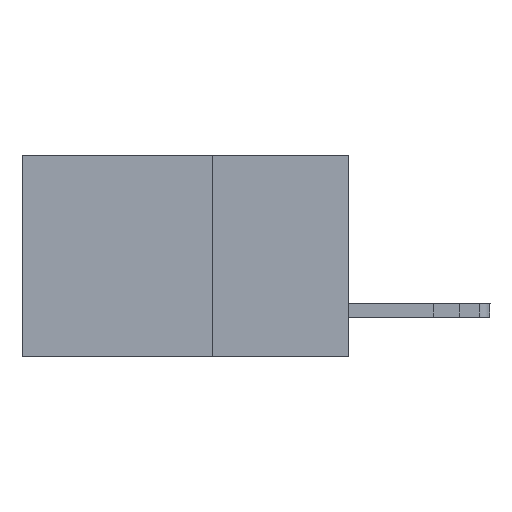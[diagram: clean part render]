
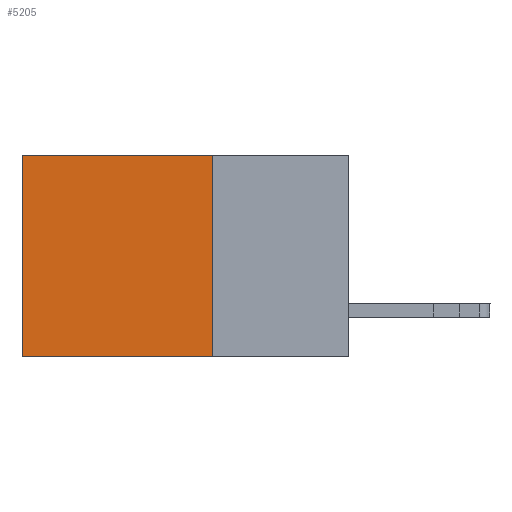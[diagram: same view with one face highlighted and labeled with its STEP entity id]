
A CAD part, left-side view. The second image highlights one B-rep face of the part: STEP entity #5205.
In plain terms, the highlighted planar face has unit normal (-1, 0, 0).
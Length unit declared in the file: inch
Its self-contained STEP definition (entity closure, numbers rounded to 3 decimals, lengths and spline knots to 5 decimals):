
#252 = EDGE_CURVE ( 'NONE', #12059, #4546, #9393, .T. ) ;
#828 = CARTESIAN_POINT ( 'NONE',  ( 0.2615, 0.25, 0. ) ) ;
#1049 = VECTOR ( 'NONE', #12565, 39.37008 ) ;
#1691 = CARTESIAN_POINT ( 'NONE',  ( 0.2615, 0.6, -0.37 ) ) ;
#1848 = EDGE_CURVE ( 'NONE', #4728, #4546, #3767, .T. ) ;
#2175 = CARTESIAN_POINT ( 'NONE',  ( 0.2615, 0.25, -0.37 ) ) ;
#2454 = CARTESIAN_POINT ( 'NONE',  ( 0.2615, 0.6, -0.37 ) ) ;
#2638 = DIRECTION ( 'NONE',  ( 0., 0., -1. ) ) ;
#3041 = CARTESIAN_POINT ( 'NONE',  ( 0.2615, 0.25, 0. ) ) ;
#3421 = VERTEX_POINT ( 'NONE', #3041 ) ;
#3476 = LINE ( 'NONE', #10399, #10697 ) ;
#3767 = LINE ( 'NONE', #2454, #10943 ) ;
#3807 = CARTESIAN_POINT ( 'NONE',  ( 0.2615, 0.6, 0. ) ) ;
#4033 = ORIENTED_EDGE ( 'NONE', *, *, #252, .F. ) ;
#4546 = VERTEX_POINT ( 'NONE', #1691 ) ;
#4728 = VERTEX_POINT ( 'NONE', #3807 ) ;
#5166 = PLANE ( 'NONE',  #7309 ) ;
#5205 = ADVANCED_FACE ( 'NONE', ( #5338 ), #5166, .F. ) ;
#5302 = DIRECTION ( 'NONE',  ( 0., 0., -1. ) ) ;
#5332 = DIRECTION ( 'NONE',  ( 1., 0., 0. ) ) ;
#5338 = FACE_OUTER_BOUND ( 'NONE', #6550, .T. ) ;
#5349 = CARTESIAN_POINT ( 'NONE',  ( 0.2615, 0.25, -0.37 ) ) ;
#6009 = EDGE_CURVE ( 'NONE', #3421, #12059, #3476, .T. ) ;
#6550 = EDGE_LOOP ( 'NONE', ( #12817, #4033, #11501, #11157 ) ) ;
#6727 = EDGE_CURVE ( 'NONE', #3421, #4728, #9016, .T. ) ;
#7309 = AXIS2_PLACEMENT_3D ( 'NONE', #5349, #5332, #5302 ) ;
#9016 = LINE ( 'NONE', #828, #1049 ) ;
#9087 = VECTOR ( 'NONE', #11078, 39.37008 ) ;
#9393 = LINE ( 'NONE', #11479, #9087 ) ;
#10177 = DIRECTION ( 'NONE',  ( 0., 0., -1. ) ) ;
#10399 = CARTESIAN_POINT ( 'NONE',  ( 0.2615, 0.25, -0.37 ) ) ;
#10697 = VECTOR ( 'NONE', #10177, 39.37008 ) ;
#10943 = VECTOR ( 'NONE', #2638, 39.37008 ) ;
#11078 = DIRECTION ( 'NONE',  ( 0., 1., 0. ) ) ;
#11157 = ORIENTED_EDGE ( 'NONE', *, *, #6727, .T. ) ;
#11479 = CARTESIAN_POINT ( 'NONE',  ( 0.2615, 0.25, -0.37 ) ) ;
#11501 = ORIENTED_EDGE ( 'NONE', *, *, #6009, .F. ) ;
#12059 = VERTEX_POINT ( 'NONE', #2175 ) ;
#12565 = DIRECTION ( 'NONE',  ( 0., 1., 0. ) ) ;
#12817 = ORIENTED_EDGE ( 'NONE', *, *, #1848, .T. ) ;
